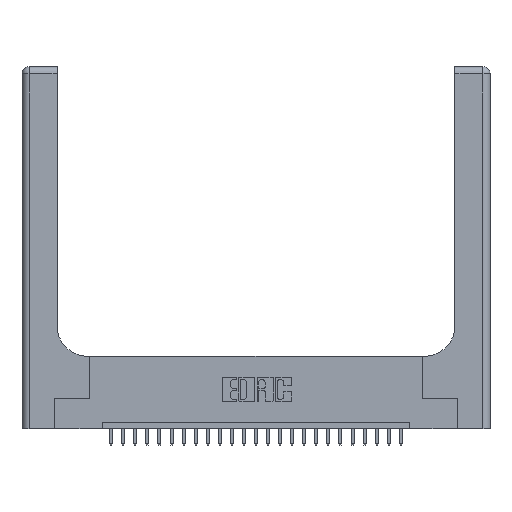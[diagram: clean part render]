
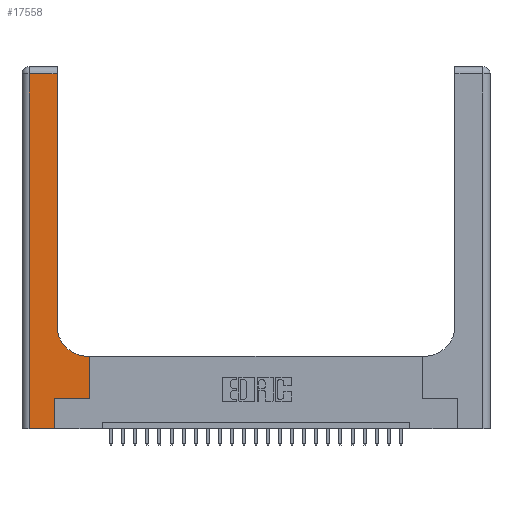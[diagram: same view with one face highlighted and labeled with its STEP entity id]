
A CAD part, top view. The second image highlights one B-rep face of the part: STEP entity #17558.
In plain terms, the highlighted planar face has unit normal (0, 0, 1).
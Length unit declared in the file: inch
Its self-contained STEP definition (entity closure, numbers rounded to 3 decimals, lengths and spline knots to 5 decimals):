
#378 = VECTOR ( 'NONE', #20637, 39.37008 ) ;
#576 = DIRECTION ( 'NONE',  ( 1., 0., 0. ) ) ;
#796 = VERTEX_POINT ( 'NONE', #5581 ) ;
#1455 = LINE ( 'NONE', #10463, #10697 ) ;
#2114 = AXIS2_PLACEMENT_3D ( 'NONE', #19212, #24964, #2904 ) ;
#2870 = CARTESIAN_POINT ( 'NONE',  ( 0.5415, 0.6, 0.37 ) ) ;
#2904 = DIRECTION ( 'NONE',  ( -1., 0., 0. ) ) ;
#3191 = CARTESIAN_POINT ( 'NONE',  ( 0.269, 0., 0.37 ) ) ;
#3545 = DIRECTION ( 'NONE',  ( 0., 1., 0. ) ) ;
#3792 = EDGE_LOOP ( 'NONE', ( #25994, #13849, #14712, #16355, #20907, #21281, #10468, #4144, #15966 ) ) ;
#3831 = CARTESIAN_POINT ( 'NONE',  ( 0.06, 2.94, 0.37 ) ) ;
#3878 = LINE ( 'NONE', #15767, #10860 ) ;
#4047 = VERTEX_POINT ( 'NONE', #17418 ) ;
#4144 = ORIENTED_EDGE ( 'NONE', *, *, #16231, .T. ) ;
#4228 = LINE ( 'NONE', #24605, #378 ) ;
#4378 = VERTEX_POINT ( 'NONE', #5459 ) ;
#4768 = VERTEX_POINT ( 'NONE', #14607 ) ;
#5017 = CARTESIAN_POINT ( 'NONE',  ( 0.2915, 0.6, 0.37 ) ) ;
#5459 = CARTESIAN_POINT ( 'NONE',  ( 0.06, 0., 0.37 ) ) ;
#5581 = CARTESIAN_POINT ( 'NONE',  ( 0.269, 0.25, 0.37 ) ) ;
#6730 = VECTOR ( 'NONE', #25579, 39.37008 ) ;
#7133 = EDGE_CURVE ( 'NONE', #9820, #11560, #20240, .T. ) ;
#7222 = DIRECTION ( 'NONE',  ( 0., 1., 0. ) ) ;
#9087 = DIRECTION ( 'NONE',  ( -1., 0., 0. ) ) ;
#9820 = VERTEX_POINT ( 'NONE', #21424 ) ;
#10463 = CARTESIAN_POINT ( 'NONE',  ( 0.269, 0.25, 0.37 ) ) ;
#10468 = ORIENTED_EDGE ( 'NONE', *, *, #24564, .T. ) ;
#10697 = VECTOR ( 'NONE', #24589, 39.37008 ) ;
#10860 = VECTOR ( 'NONE', #3545, 39.37008 ) ;
#11346 = CARTESIAN_POINT ( 'NONE',  ( 0.5585, 0.25, 0.37 ) ) ;
#11560 = VERTEX_POINT ( 'NONE', #3831 ) ;
#12128 = LINE ( 'NONE', #11346, #6730 ) ;
#13297 = VECTOR ( 'NONE', #9087, 39.37008 ) ;
#13400 = EDGE_CURVE ( 'NONE', #4378, #18998, #4228, .T. ) ;
#13511 = EDGE_CURVE ( 'NONE', #24922, #4768, #21381, .T. ) ;
#13849 = ORIENTED_EDGE ( 'NONE', *, *, #7133, .T. ) ;
#14059 = EDGE_CURVE ( 'NONE', #4768, #9820, #3878, .T. ) ;
#14101 = VERTEX_POINT ( 'NONE', #25435 ) ;
#14173 = FACE_OUTER_BOUND ( 'NONE', #3792, .T. ) ;
#14607 = CARTESIAN_POINT ( 'NONE',  ( 0.2915, 0.85, 0.37 ) ) ;
#14706 = DIRECTION ( 'NONE',  ( 0., 0., -1. ) ) ;
#14712 = ORIENTED_EDGE ( 'NONE', *, *, #24178, .T. ) ;
#15767 = CARTESIAN_POINT ( 'NONE',  ( 0.2915, 3., 0.37 ) ) ;
#15891 = LINE ( 'NONE', #16092, #19717 ) ;
#15957 = CARTESIAN_POINT ( 'NONE',  ( 0.269, 0., 0.37 ) ) ;
#15966 = ORIENTED_EDGE ( 'NONE', *, *, #13511, .T. ) ;
#16092 = CARTESIAN_POINT ( 'NONE',  ( 0.06, 3., 0.37 ) ) ;
#16138 = LINE ( 'NONE', #5017, #13297 ) ;
#16231 = EDGE_CURVE ( 'NONE', #4047, #24922, #16138, .T. ) ;
#16355 = ORIENTED_EDGE ( 'NONE', *, *, #13400, .T. ) ;
#16837 = CARTESIAN_POINT ( 'NONE',  ( 0., 2.94, 0.37 ) ) ;
#17411 = VECTOR ( 'NONE', #19691, 39.37008 ) ;
#17418 = CARTESIAN_POINT ( 'NONE',  ( 0.5585, 0.6, 0.37 ) ) ;
#17558 = ADVANCED_FACE ( 'NONE', ( #14173 ), #22592, .F. ) ;
#18998 = VERTEX_POINT ( 'NONE', #15957 ) ;
#19212 = CARTESIAN_POINT ( 'NONE',  ( 0., 3., 0.37 ) ) ;
#19427 = AXIS2_PLACEMENT_3D ( 'NONE', #25056, #14706, #576 ) ;
#19691 = DIRECTION ( 'NONE',  ( -1., 0., 0. ) ) ;
#19717 = VECTOR ( 'NONE', #25925, 39.37008 ) ;
#20240 = LINE ( 'NONE', #16837, #17411 ) ;
#20637 = DIRECTION ( 'NONE',  ( 1., 0., 0. ) ) ;
#20907 = ORIENTED_EDGE ( 'NONE', *, *, #22341, .T. ) ;
#21073 = EDGE_CURVE ( 'NONE', #796, #14101, #1455, .T. ) ;
#21281 = ORIENTED_EDGE ( 'NONE', *, *, #21073, .T. ) ;
#21381 = CIRCLE ( 'NONE', #19427, 0.25 ) ;
#21424 = CARTESIAN_POINT ( 'NONE',  ( 0.2915, 2.94, 0.37 ) ) ;
#22341 = EDGE_CURVE ( 'NONE', #18998, #796, #24219, .T. ) ;
#22592 = PLANE ( 'NONE',  #2114 ) ;
#24178 = EDGE_CURVE ( 'NONE', #11560, #4378, #15891, .T. ) ;
#24219 = LINE ( 'NONE', #3191, #25505 ) ;
#24564 = EDGE_CURVE ( 'NONE', #14101, #4047, #12128, .T. ) ;
#24589 = DIRECTION ( 'NONE',  ( 1., 0., 0. ) ) ;
#24605 = CARTESIAN_POINT ( 'NONE',  ( 0., 0., 0.37 ) ) ;
#24922 = VERTEX_POINT ( 'NONE', #2870 ) ;
#24964 = DIRECTION ( 'NONE',  ( 0., 0., -1. ) ) ;
#25056 = CARTESIAN_POINT ( 'NONE',  ( 0.5415, 0.85, 0.37 ) ) ;
#25435 = CARTESIAN_POINT ( 'NONE',  ( 0.5585, 0.25, 0.37 ) ) ;
#25505 = VECTOR ( 'NONE', #7222, 39.37008 ) ;
#25579 = DIRECTION ( 'NONE',  ( 0., 1., 0. ) ) ;
#25925 = DIRECTION ( 'NONE',  ( 0., -1., 0. ) ) ;
#25994 = ORIENTED_EDGE ( 'NONE', *, *, #14059, .T. ) ;
